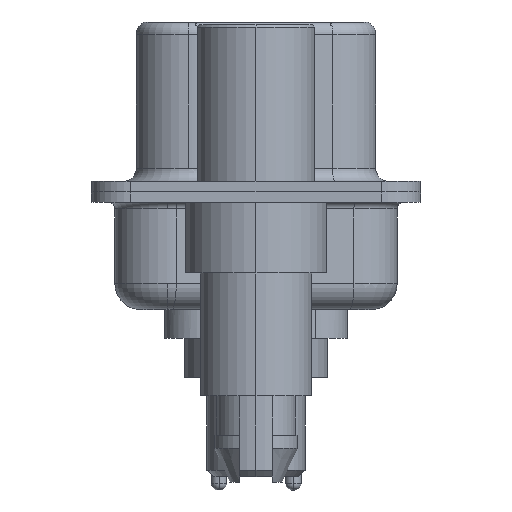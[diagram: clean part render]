
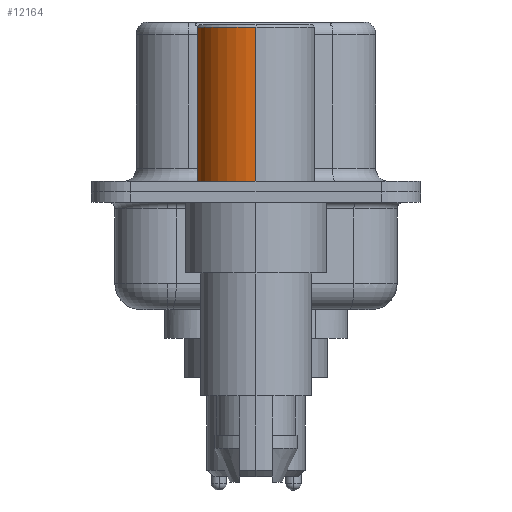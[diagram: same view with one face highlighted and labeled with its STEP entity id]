
A CAD part, left-side view. The second image highlights one B-rep face of the part: STEP entity #12164.
In plain terms, the highlighted cylindrical face has radius 2.25 mm (diameter 4.5 mm), a partial arc.
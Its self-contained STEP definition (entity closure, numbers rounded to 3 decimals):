
#438 = VERTEX_POINT ( 'NONE', #10918 ) ;
#2228 = AXIS2_PLACEMENT_3D ( 'NONE', #2369, #21566, #19907 ) ;
#2369 = CARTESIAN_POINT ( 'NONE',  ( 0., 0., 0.581 ) ) ;
#2656 = DIRECTION ( 'NONE',  ( 1., 0., 0. ) ) ;
#3541 = LINE ( 'NONE', #10464, #21070 ) ;
#3643 = VECTOR ( 'NONE', #20011, 1000. ) ;
#3730 = VERTEX_POINT ( 'NONE', #13654 ) ;
#3847 = EDGE_CURVE ( 'NONE', #11304, #3730, #20624, .T. ) ;
#5448 = ORIENTED_EDGE ( 'NONE', *, *, #3847, .F. ) ;
#5566 = CIRCLE ( 'NONE', #12387, 2.25 ) ;
#6770 = EDGE_CURVE ( 'NONE', #17628, #3730, #3541, .T. ) ;
#7656 = EDGE_LOOP ( 'NONE', ( #15958, #14848, #5448, #22675 ) ) ;
#7729 = CARTESIAN_POINT ( 'NONE',  ( 2.25, 0., 0.581 ) ) ;
#8125 = CARTESIAN_POINT ( 'NONE',  ( -2.25, 0., 0.4 ) ) ;
#8294 = CYLINDRICAL_SURFACE ( 'NONE', #2228, 2.25 ) ;
#9632 = CARTESIAN_POINT ( 'NONE',  ( 0., 0., 0.4 ) ) ;
#10464 = CARTESIAN_POINT ( 'NONE',  ( -2.25, 0., 0.581 ) ) ;
#10918 = CARTESIAN_POINT ( 'NONE',  ( 2.25, 0., 0.4 ) ) ;
#11182 = CARTESIAN_POINT ( 'NONE',  ( 2.25, 0., 6.3 ) ) ;
#11304 = VERTEX_POINT ( 'NONE', #11182 ) ;
#11958 = AXIS2_PLACEMENT_3D ( 'NONE', #20861, #22636, #13975 ) ;
#12164 = ADVANCED_FACE ( 'NONE', ( #20634 ), #8294, .T. ) ;
#12266 = DIRECTION ( 'NONE',  ( 0., 0., 1. ) ) ;
#12296 = EDGE_CURVE ( 'NONE', #438, #17628, #5566, .T. ) ;
#12387 = AXIS2_PLACEMENT_3D ( 'NONE', #9632, #13200, #2656 ) ;
#13110 = EDGE_CURVE ( 'NONE', #438, #11304, #15468, .T. ) ;
#13200 = DIRECTION ( 'NONE',  ( 0., 0., 1. ) ) ;
#13654 = CARTESIAN_POINT ( 'NONE',  ( -2.25, 0., 6.3 ) ) ;
#13975 = DIRECTION ( 'NONE',  ( 1., 0., 0. ) ) ;
#14848 = ORIENTED_EDGE ( 'NONE', *, *, #6770, .T. ) ;
#15468 = LINE ( 'NONE', #7729, #3643 ) ;
#15958 = ORIENTED_EDGE ( 'NONE', *, *, #12296, .T. ) ;
#17628 = VERTEX_POINT ( 'NONE', #8125 ) ;
#19907 = DIRECTION ( 'NONE',  ( 1., 0., 0. ) ) ;
#20011 = DIRECTION ( 'NONE',  ( 0., 0., 1. ) ) ;
#20624 = CIRCLE ( 'NONE', #11958, 2.25 ) ;
#20634 = FACE_OUTER_BOUND ( 'NONE', #7656, .T. ) ;
#20861 = CARTESIAN_POINT ( 'NONE',  ( 0., 0., 6.3 ) ) ;
#21070 = VECTOR ( 'NONE', #12266, 1000. ) ;
#21566 = DIRECTION ( 'NONE',  ( 0., 0., 1. ) ) ;
#22636 = DIRECTION ( 'NONE',  ( 0., 0., 1. ) ) ;
#22675 = ORIENTED_EDGE ( 'NONE', *, *, #13110, .F. ) ;
